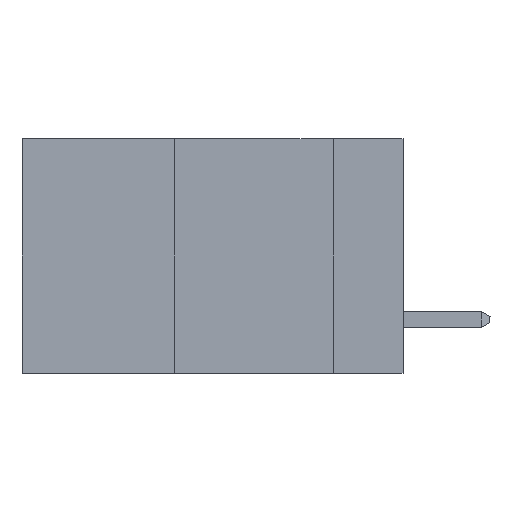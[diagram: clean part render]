
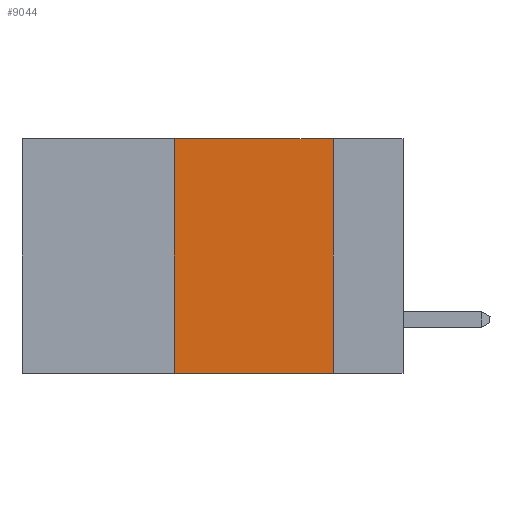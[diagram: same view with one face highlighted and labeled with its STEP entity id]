
A CAD part, left-side view. The second image highlights one B-rep face of the part: STEP entity #9044.
In plain terms, the highlighted planar face has unit normal (-1, 0, 0).
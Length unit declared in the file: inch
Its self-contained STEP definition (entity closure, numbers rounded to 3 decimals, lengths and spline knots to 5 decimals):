
#64 = PLANE ( 'NONE',  #8617 ) ;
#390 = DIRECTION ( 'NONE',  ( 0., -1., 0. ) ) ;
#520 = VECTOR ( 'NONE', #390, 39.37008 ) ;
#2493 = ORIENTED_EDGE ( 'NONE', *, *, #14300, .F. ) ;
#3030 = LINE ( 'NONE', #20211, #19561 ) ;
#3105 = ORIENTED_EDGE ( 'NONE', *, *, #23643, .T. ) ;
#4516 = CARTESIAN_POINT ( 'NONE',  ( 0., 0.6, 0. ) ) ;
#5025 = VECTOR ( 'NONE', #17823, 39.37008 ) ;
#5797 = ORIENTED_EDGE ( 'NONE', *, *, #11843, .F. ) ;
#6055 = CARTESIAN_POINT ( 'NONE',  ( 0., 0.36, -0.37 ) ) ;
#7707 = DIRECTION ( 'NONE',  ( 1., 0., 0. ) ) ;
#7912 = EDGE_LOOP ( 'NONE', ( #5797, #9046, #2493, #3105 ) ) ;
#8068 = CARTESIAN_POINT ( 'NONE',  ( 0., 0.36, 0. ) ) ;
#8617 = AXIS2_PLACEMENT_3D ( 'NONE', #22877, #7707, #17119 ) ;
#9044 = ADVANCED_FACE ( 'NONE', ( #9475 ), #64, .F. ) ;
#9046 = ORIENTED_EDGE ( 'NONE', *, *, #10368, .F. ) ;
#9475 = FACE_OUTER_BOUND ( 'NONE', #7912, .T. ) ;
#9953 = CARTESIAN_POINT ( 'NONE',  ( 0., 0.11, 0. ) ) ;
#10209 = LINE ( 'NONE', #15848, #19086 ) ;
#10368 = EDGE_CURVE ( 'NONE', #15437, #11654, #21702, .T. ) ;
#11654 = VERTEX_POINT ( 'NONE', #9953 ) ;
#11843 = EDGE_CURVE ( 'NONE', #11654, #17584, #10209, .T. ) ;
#14300 = EDGE_CURVE ( 'NONE', #22015, #15437, #3030, .T. ) ;
#14320 = DIRECTION ( 'NONE',  ( 0., 0., -1. ) ) ;
#14500 = CARTESIAN_POINT ( 'NONE',  ( 0., 0.11, -0.37 ) ) ;
#15437 = VERTEX_POINT ( 'NONE', #8068 ) ;
#15848 = CARTESIAN_POINT ( 'NONE',  ( 0., 0.11, 0. ) ) ;
#16438 = DIRECTION ( 'NONE',  ( 0., 0., 1. ) ) ;
#17119 = DIRECTION ( 'NONE',  ( 0., 0., -1. ) ) ;
#17584 = VERTEX_POINT ( 'NONE', #14500 ) ;
#17689 = LINE ( 'NONE', #20944, #520 ) ;
#17823 = DIRECTION ( 'NONE',  ( 0., -1., 0. ) ) ;
#19086 = VECTOR ( 'NONE', #14320, 39.37008 ) ;
#19561 = VECTOR ( 'NONE', #16438, 39.37008 ) ;
#20211 = CARTESIAN_POINT ( 'NONE',  ( 0., 0.36, 0. ) ) ;
#20944 = CARTESIAN_POINT ( 'NONE',  ( 0., 0.6, -0.37 ) ) ;
#21702 = LINE ( 'NONE', #4516, #5025 ) ;
#22015 = VERTEX_POINT ( 'NONE', #6055 ) ;
#22877 = CARTESIAN_POINT ( 'NONE',  ( 0., 0.6, 0. ) ) ;
#23643 = EDGE_CURVE ( 'NONE', #22015, #17584, #17689, .T. ) ;
